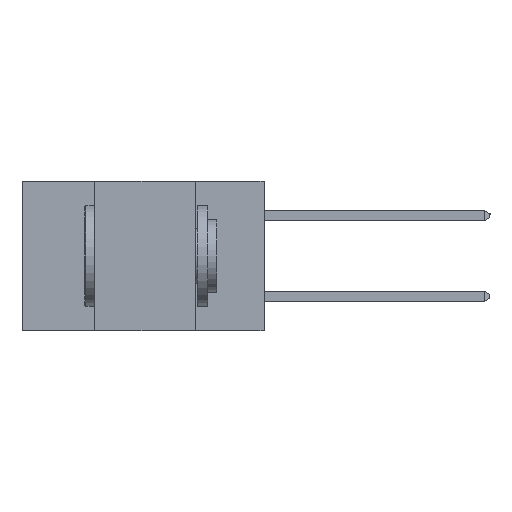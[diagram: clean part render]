
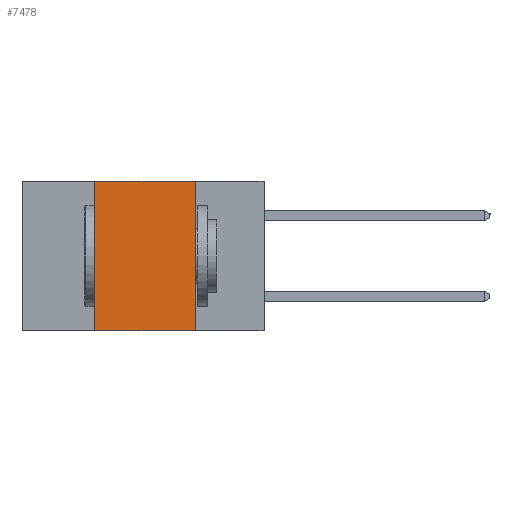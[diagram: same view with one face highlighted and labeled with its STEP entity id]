
A CAD part, left-side view. The second image highlights one B-rep face of the part: STEP entity #7478.
In plain terms, the highlighted planar face has unit normal (-1, 0, 0).
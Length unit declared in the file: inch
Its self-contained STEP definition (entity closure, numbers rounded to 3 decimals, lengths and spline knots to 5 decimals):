
#678 = LINE ( 'NONE', #8631, #12417 ) ;
#2918 = DIRECTION ( 'NONE',  ( 0., -1., 0. ) ) ;
#3961 = CARTESIAN_POINT ( 'NONE',  ( 0., 0.17, -0.37 ) ) ;
#4770 = CARTESIAN_POINT ( 'NONE',  ( 0., 0.42, -0.37 ) ) ;
#6268 = EDGE_CURVE ( 'NONE', #14659, #22890, #18677, .T. ) ;
#6284 = ORIENTED_EDGE ( 'NONE', *, *, #21097, .F. ) ;
#7478 = ADVANCED_FACE ( 'NONE', ( #17109 ), #14721, .F. ) ;
#8073 = VERTEX_POINT ( 'NONE', #9304 ) ;
#8127 = EDGE_CURVE ( 'NONE', #8073, #22890, #21464, .T. ) ;
#8631 = CARTESIAN_POINT ( 'NONE',  ( 0., 0.6, 0. ) ) ;
#9244 = CARTESIAN_POINT ( 'NONE',  ( 0., 0.17, -0.37 ) ) ;
#9304 = CARTESIAN_POINT ( 'NONE',  ( 0., 0.42, -0.37 ) ) ;
#9446 = ORIENTED_EDGE ( 'NONE', *, *, #8127, .T. ) ;
#9923 = VERTEX_POINT ( 'NONE', #25371 ) ;
#11423 = ORIENTED_EDGE ( 'NONE', *, *, #24528, .F. ) ;
#12417 = VECTOR ( 'NONE', #2918, 39.37008 ) ;
#12474 = LINE ( 'NONE', #4770, #19858 ) ;
#13018 = VECTOR ( 'NONE', #19772, 39.37008 ) ;
#13186 = CARTESIAN_POINT ( 'NONE',  ( 0., 0.17, 0. ) ) ;
#14602 = DIRECTION ( 'NONE',  ( 0., 0., -1. ) ) ;
#14659 = VERTEX_POINT ( 'NONE', #13186 ) ;
#14721 = PLANE ( 'NONE',  #20448 ) ;
#16780 = EDGE_LOOP ( 'NONE', ( #21757, #11423, #6284, #9446 ) ) ;
#16927 = DIRECTION ( 'NONE',  ( 0., 0., 1. ) ) ;
#17109 = FACE_OUTER_BOUND ( 'NONE', #16780, .T. ) ;
#18677 = LINE ( 'NONE', #9244, #19475 ) ;
#19475 = VECTOR ( 'NONE', #23246, 39.37008 ) ;
#19772 = DIRECTION ( 'NONE',  ( 0., -1., 0. ) ) ;
#19858 = VECTOR ( 'NONE', #16927, 39.37008 ) ;
#19906 = CARTESIAN_POINT ( 'NONE',  ( 0., 0.6, -0.37 ) ) ;
#20448 = AXIS2_PLACEMENT_3D ( 'NONE', #20896, #22708, #14602 ) ;
#20896 = CARTESIAN_POINT ( 'NONE',  ( 0., 0.6, 0. ) ) ;
#21097 = EDGE_CURVE ( 'NONE', #8073, #9923, #12474, .T. ) ;
#21464 = LINE ( 'NONE', #19906, #13018 ) ;
#21757 = ORIENTED_EDGE ( 'NONE', *, *, #6268, .F. ) ;
#22708 = DIRECTION ( 'NONE',  ( 1., 0., 0. ) ) ;
#22890 = VERTEX_POINT ( 'NONE', #3961 ) ;
#23246 = DIRECTION ( 'NONE',  ( 0., 0., -1. ) ) ;
#24528 = EDGE_CURVE ( 'NONE', #9923, #14659, #678, .T. ) ;
#25371 = CARTESIAN_POINT ( 'NONE',  ( 0., 0.42, 0. ) ) ;
